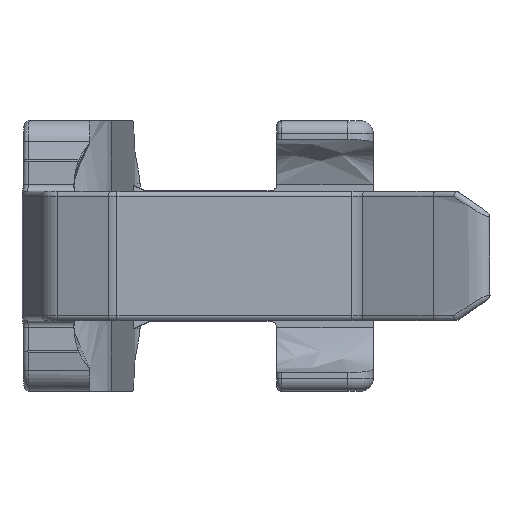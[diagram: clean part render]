
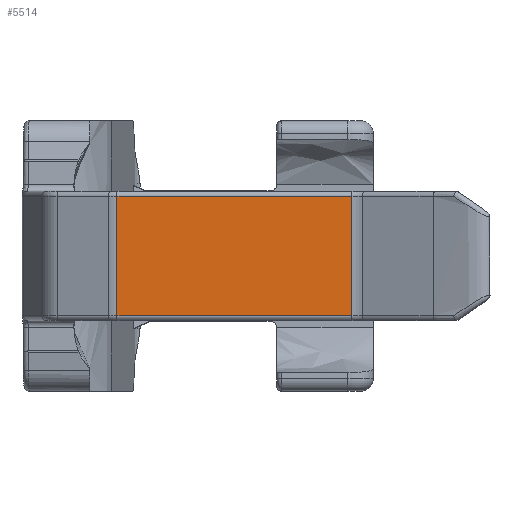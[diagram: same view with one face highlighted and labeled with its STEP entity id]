
A CAD part, left-side view. The second image highlights one B-rep face of the part: STEP entity #5514.
In plain terms, the highlighted planar face has unit normal (-1, 0, 0).
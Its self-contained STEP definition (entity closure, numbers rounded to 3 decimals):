
#248 = EDGE_CURVE ( 'NONE', #3923, #2038, #4025, .T. ) ;
#541 = ORIENTED_EDGE ( 'NONE', *, *, #248, .T. ) ;
#687 = CARTESIAN_POINT ( 'NONE',  ( -36.507, 2.923, 15.35 ) ) ;
#785 = CARTESIAN_POINT ( 'NONE',  ( -36.507, 21.423, 5.95 ) ) ;
#1202 = CARTESIAN_POINT ( 'NONE',  ( -36.507, 2.923, 0. ) ) ;
#1237 = LINE ( 'NONE', #2166, #2655 ) ;
#1268 = VECTOR ( 'NONE', #1862, 1000. ) ;
#1612 = EDGE_LOOP ( 'NONE', ( #2673, #5942, #541, #4926 ) ) ;
#1640 = DIRECTION ( 'NONE',  ( 0., -1., 0. ) ) ;
#1862 = DIRECTION ( 'NONE',  ( 0., 1., 0. ) ) ;
#1993 = VERTEX_POINT ( 'NONE', #785 ) ;
#2038 = VERTEX_POINT ( 'NONE', #687 ) ;
#2071 = PLANE ( 'NONE',  #2454 ) ;
#2155 = DIRECTION ( 'NONE',  ( 0., 0., 1. ) ) ;
#2166 = CARTESIAN_POINT ( 'NONE',  ( -36.507, 21.423, 0. ) ) ;
#2188 = EDGE_CURVE ( 'NONE', #2038, #4167, #3639, .T. ) ;
#2452 = EDGE_CURVE ( 'NONE', #1993, #4167, #1237, .T. ) ;
#2454 = AXIS2_PLACEMENT_3D ( 'NONE', #1202, #3090, #5011 ) ;
#2547 = VECTOR ( 'NONE', #1640, 1000. ) ;
#2655 = VECTOR ( 'NONE', #3095, 1000. ) ;
#2673 = ORIENTED_EDGE ( 'NONE', *, *, #2452, .F. ) ;
#2782 = VECTOR ( 'NONE', #2155, 1000. ) ;
#3017 = LINE ( 'NONE', #5882, #2547 ) ;
#3090 = DIRECTION ( 'NONE',  ( 1., 0., 0. ) ) ;
#3095 = DIRECTION ( 'NONE',  ( 0., 0., 1. ) ) ;
#3639 = LINE ( 'NONE', #4231, #1268 ) ;
#3923 = VERTEX_POINT ( 'NONE', #4643 ) ;
#4025 = LINE ( 'NONE', #4119, #2782 ) ;
#4119 = CARTESIAN_POINT ( 'NONE',  ( -36.507, 2.923, 0. ) ) ;
#4167 = VERTEX_POINT ( 'NONE', #5354 ) ;
#4231 = CARTESIAN_POINT ( 'NONE',  ( -36.507, 21.423, 15.35 ) ) ;
#4643 = CARTESIAN_POINT ( 'NONE',  ( -36.507, 2.923, 5.95 ) ) ;
#4926 = ORIENTED_EDGE ( 'NONE', *, *, #2188, .T. ) ;
#5011 = DIRECTION ( 'NONE',  ( 0., -1., 0. ) ) ;
#5354 = CARTESIAN_POINT ( 'NONE',  ( -36.507, 21.423, 15.35 ) ) ;
#5428 = FACE_OUTER_BOUND ( 'NONE', #1612, .T. ) ;
#5514 = ADVANCED_FACE ( 'NONE', ( #5428 ), #2071, .F. ) ;
#5525 = EDGE_CURVE ( 'NONE', #1993, #3923, #3017, .T. ) ;
#5882 = CARTESIAN_POINT ( 'NONE',  ( -36.507, 2.923, 5.95 ) ) ;
#5942 = ORIENTED_EDGE ( 'NONE', *, *, #5525, .T. ) ;
